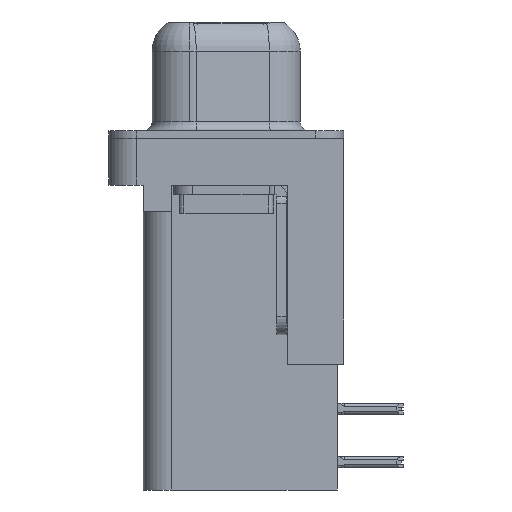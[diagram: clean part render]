
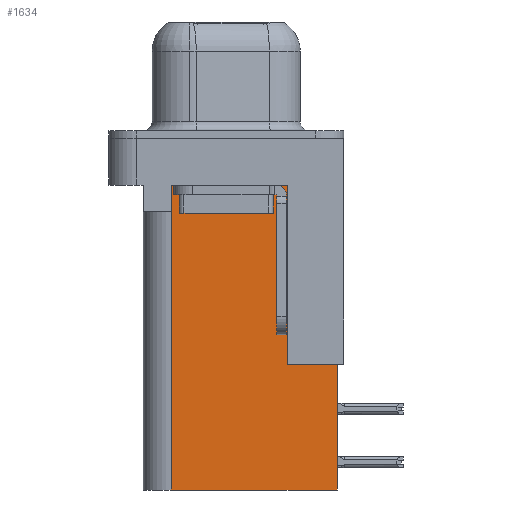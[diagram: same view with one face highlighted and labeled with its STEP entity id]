
A CAD part, left-side view. The second image highlights one B-rep face of the part: STEP entity #1634.
In plain terms, the highlighted planar face has unit normal (-1, 0, 0).
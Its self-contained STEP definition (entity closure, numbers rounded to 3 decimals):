
#442 = ORIENTED_EDGE ( 'NONE', *, *, #6566, .F. ) ;
#460 = VERTEX_POINT ( 'NONE', #20539 ) ;
#728 = DIRECTION ( 'NONE',  ( 0., 1., 0. ) ) ;
#852 = DIRECTION ( 'NONE',  ( 0., 1., 0. ) ) ;
#966 = EDGE_CURVE ( 'NONE', #3672, #21892, #5008, .T. ) ;
#1634 = ADVANCED_FACE ( 'NONE', ( #2446 ), #11283, .F. ) ;
#2446 = FACE_OUTER_BOUND ( 'NONE', #13813, .T. ) ;
#2497 = LINE ( 'NONE', #16201, #10795 ) ;
#2583 = EDGE_CURVE ( 'NONE', #7408, #16933, #7323, .T. ) ;
#3155 = CARTESIAN_POINT ( 'NONE',  ( 3.79, -5.925, -2. ) ) ;
#3156 = CARTESIAN_POINT ( 'NONE',  ( 3.79, -3.295, -18.76 ) ) ;
#3283 = CARTESIAN_POINT ( 'NONE',  ( 3.79, -3.295, -18.76 ) ) ;
#3672 = VERTEX_POINT ( 'NONE', #3801 ) ;
#3801 = CARTESIAN_POINT ( 'NONE',  ( 3.79, 2.895, -3.9 ) ) ;
#4919 = EDGE_CURVE ( 'NONE', #9787, #21892, #19996, .T. ) ;
#5008 = LINE ( 'NONE', #7150, #13227 ) ;
#5091 = DIRECTION ( 'NONE',  ( 0., 1., 0. ) ) ;
#6496 = CARTESIAN_POINT ( 'NONE',  ( 3.79, 2.925, -18.76 ) ) ;
#6566 = EDGE_CURVE ( 'NONE', #8629, #9787, #16338, .T. ) ;
#7150 = CARTESIAN_POINT ( 'NONE',  ( 3.79, 0., -3.9 ) ) ;
#7276 = ORIENTED_EDGE ( 'NONE', *, *, #10814, .T. ) ;
#7323 = LINE ( 'NONE', #25141, #22490 ) ;
#7408 = VERTEX_POINT ( 'NONE', #24036 ) ;
#8514 = DIRECTION ( 'NONE',  ( 0., 0., 1. ) ) ;
#8629 = VERTEX_POINT ( 'NONE', #20970 ) ;
#9137 = ORIENTED_EDGE ( 'NONE', *, *, #2583, .T. ) ;
#9787 = VERTEX_POINT ( 'NONE', #10544 ) ;
#9991 = VECTOR ( 'NONE', #728, 1000. ) ;
#10332 = CARTESIAN_POINT ( 'NONE',  ( 3.79, 2.925, -3.9 ) ) ;
#10544 = CARTESIAN_POINT ( 'NONE',  ( 3.79, 2.925, -18.76 ) ) ;
#10795 = VECTOR ( 'NONE', #18193, 1000. ) ;
#10814 = EDGE_CURVE ( 'NONE', #20146, #7408, #13532, .T. ) ;
#11283 = PLANE ( 'NONE',  #16032 ) ;
#12646 = DIRECTION ( 'NONE',  ( 1., 0., 0. ) ) ;
#12954 = ORIENTED_EDGE ( 'NONE', *, *, #966, .T. ) ;
#13227 = VECTOR ( 'NONE', #22665, 1000. ) ;
#13532 = LINE ( 'NONE', #3283, #14354 ) ;
#13812 = EDGE_CURVE ( 'NONE', #16933, #3672, #2497, .T. ) ;
#13813 = EDGE_LOOP ( 'NONE', ( #9137, #15035, #12954, #22634, #442, #22707, #18020, #7276 ) ) ;
#14354 = VECTOR ( 'NONE', #17289, 1000. ) ;
#14929 = EDGE_CURVE ( 'NONE', #460, #20146, #18252, .T. ) ;
#15035 = ORIENTED_EDGE ( 'NONE', *, *, #13812, .T. ) ;
#15163 = EDGE_CURVE ( 'NONE', #460, #8629, #22492, .T. ) ;
#16032 = AXIS2_PLACEMENT_3D ( 'NONE', #18447, #12646, #852 ) ;
#16201 = CARTESIAN_POINT ( 'NONE',  ( 3.79, 2.895, -3.9 ) ) ;
#16338 = LINE ( 'NONE', #3156, #22271 ) ;
#16933 = VERTEX_POINT ( 'NONE', #23482 ) ;
#17160 = DIRECTION ( 'NONE',  ( 0., 0., -1. ) ) ;
#17289 = DIRECTION ( 'NONE',  ( 0., 0., 1. ) ) ;
#18020 = ORIENTED_EDGE ( 'NONE', *, *, #14929, .T. ) ;
#18148 = VECTOR ( 'NONE', #17160, 1000. ) ;
#18193 = DIRECTION ( 'NONE',  ( 0., 0., -1. ) ) ;
#18252 = LINE ( 'NONE', #18489, #9991 ) ;
#18447 = CARTESIAN_POINT ( 'NONE',  ( 3.79, -3.295, -18.76 ) ) ;
#18489 = CARTESIAN_POINT ( 'NONE',  ( 3.79, -6.295, -12.05 ) ) ;
#18616 = CARTESIAN_POINT ( 'NONE',  ( 3.79, -3.295, -12.05 ) ) ;
#19996 = LINE ( 'NONE', #6496, #20048 ) ;
#20048 = VECTOR ( 'NONE', #8514, 1000. ) ;
#20146 = VERTEX_POINT ( 'NONE', #18616 ) ;
#20539 = CARTESIAN_POINT ( 'NONE',  ( 3.79, -5.925, -12.05 ) ) ;
#20970 = CARTESIAN_POINT ( 'NONE',  ( 3.79, -5.925, -18.76 ) ) ;
#21892 = VERTEX_POINT ( 'NONE', #10332 ) ;
#22271 = VECTOR ( 'NONE', #5091, 1000. ) ;
#22490 = VECTOR ( 'NONE', #25229, 1000. ) ;
#22492 = LINE ( 'NONE', #3155, #18148 ) ;
#22634 = ORIENTED_EDGE ( 'NONE', *, *, #4919, .F. ) ;
#22665 = DIRECTION ( 'NONE',  ( 0., 1., 0. ) ) ;
#22707 = ORIENTED_EDGE ( 'NONE', *, *, #15163, .F. ) ;
#23482 = CARTESIAN_POINT ( 'NONE',  ( 3.79, 2.895, -2.5 ) ) ;
#24036 = CARTESIAN_POINT ( 'NONE',  ( 3.79, -3.295, -2.5 ) ) ;
#25141 = CARTESIAN_POINT ( 'NONE',  ( 3.79, -3.295, -2.5 ) ) ;
#25229 = DIRECTION ( 'NONE',  ( 0., 1., 0. ) ) ;
